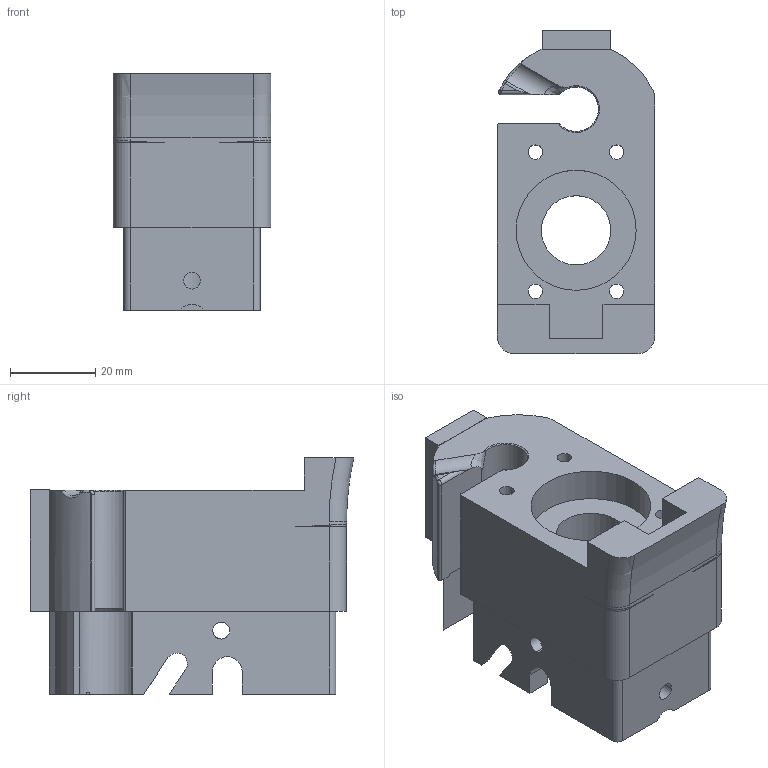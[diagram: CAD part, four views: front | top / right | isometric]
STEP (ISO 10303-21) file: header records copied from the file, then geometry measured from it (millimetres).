
FILE_DESCRIPTION(/* description */ (''),/* implementation_level */ '2;1');
FILE_NAME(/* name */ 'Barrel Retainer.step',/* time_stamp */ '2022-05-11T21:15:34-06:00',/* author */ (''),/* organization */ (''),/* preprocessor_version */ 'ST-DEVELOPER v18.1',/* originating_system */ 'Autodesk Translation Framework v10.10.0.1391',/* authorisation */ '');
FILE_SCHEMA (('AUTOMOTIVE_DESIGN { 1 0 10303 214 3 1 1 }'));
Length unit declared in the file: millimetre
Products named in the file (1): Barrel Retainer (1)
Bounding box: 37.08 x 76.18 x 55.65 mm (x, y, z)
Volume: 63265 mm3; surface area: 23350.8 mm2
Topology: 1 solids, 1 shells, 181 faces, 511 edges, 331 vertices
Faces by surface type: plane 95, cylinder 62, bspline 19, torus 4, cone 1
Full cylindrical faces by diameter (mm): 2.65 x1, 3 x1, 3.4 x4, 4 x4, 4.5 x1, 16.3 x1, 28.25 x1
Entity records: 6813 total; most frequent: CARTESIAN_POINT 2145, ORIENTED_EDGE 1006, DIRECTION 908, EDGE_CURVE 503, VERTEX_POINT 331, LINE 304, VECTOR 304, AXIS2_PLACEMENT_3D 302
